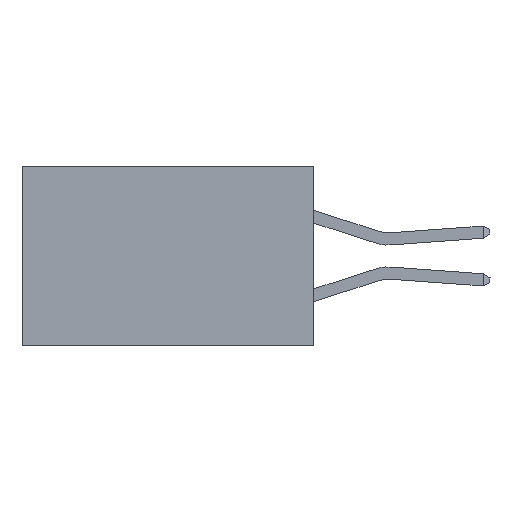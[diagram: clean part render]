
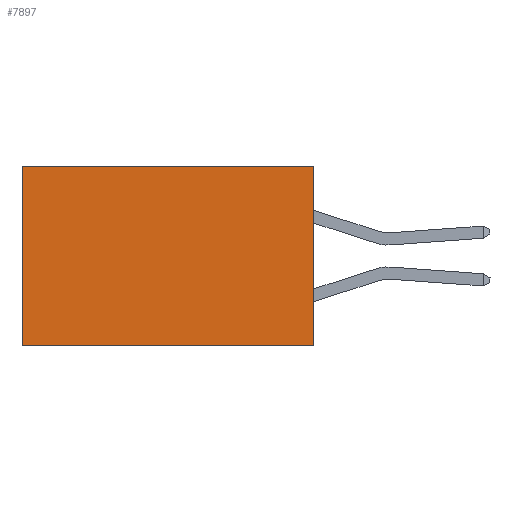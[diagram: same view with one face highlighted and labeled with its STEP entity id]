
A CAD part, left-side view. The second image highlights one B-rep face of the part: STEP entity #7897.
In plain terms, the highlighted planar face has unit normal (-1, 0, 0).
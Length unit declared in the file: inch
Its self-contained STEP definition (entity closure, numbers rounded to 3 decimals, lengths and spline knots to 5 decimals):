
#420 = VECTOR ( 'NONE', #7155, 39.37008 ) ;
#629 = CARTESIAN_POINT ( 'NONE',  ( 0.2875, 0., -0.37 ) ) ;
#686 = VERTEX_POINT ( 'NONE', #1761 ) ;
#1224 = ORIENTED_EDGE ( 'NONE', *, *, #5852, .F. ) ;
#1421 = EDGE_CURVE ( 'NONE', #686, #5934, #5172, .T. ) ;
#1761 = CARTESIAN_POINT ( 'NONE',  ( 0.2875, 0., 0. ) ) ;
#1765 = CARTESIAN_POINT ( 'NONE',  ( 0.2875, 0., 0. ) ) ;
#2211 = CARTESIAN_POINT ( 'NONE',  ( 0.2875, 0.6, -0.37 ) ) ;
#2375 = LINE ( 'NONE', #3022, #420 ) ;
#2548 = ORIENTED_EDGE ( 'NONE', *, *, #4439, .F. ) ;
#2642 = VERTEX_POINT ( 'NONE', #2211 ) ;
#2673 = ORIENTED_EDGE ( 'NONE', *, *, #1421, .T. ) ;
#2735 = AXIS2_PLACEMENT_3D ( 'NONE', #5679, #3637, #8225 ) ;
#2914 = FACE_OUTER_BOUND ( 'NONE', #3984, .T. ) ;
#2983 = PLANE ( 'NONE',  #2735 ) ;
#3022 = CARTESIAN_POINT ( 'NONE',  ( 0.2875, 0., -0.37 ) ) ;
#3075 = VECTOR ( 'NONE', #8655, 39.37008 ) ;
#3130 = CARTESIAN_POINT ( 'NONE',  ( 0.2875, 0.6, 0. ) ) ;
#3423 = ORIENTED_EDGE ( 'NONE', *, *, #3440, .T. ) ;
#3433 = DIRECTION ( 'NONE',  ( 0., 1., 0. ) ) ;
#3440 = EDGE_CURVE ( 'NONE', #5934, #2642, #6630, .T. ) ;
#3637 = DIRECTION ( 'NONE',  ( 1., 0., 0. ) ) ;
#3667 = LINE ( 'NONE', #6379, #5019 ) ;
#3984 = EDGE_LOOP ( 'NONE', ( #3423, #1224, #2548, #2673 ) ) ;
#4439 = EDGE_CURVE ( 'NONE', #686, #5894, #3667, .T. ) ;
#5019 = VECTOR ( 'NONE', #8525, 39.37008 ) ;
#5172 = LINE ( 'NONE', #1765, #6987 ) ;
#5679 = CARTESIAN_POINT ( 'NONE',  ( 0.2875, 0., 0. ) ) ;
#5852 = EDGE_CURVE ( 'NONE', #5894, #2642, #2375, .T. ) ;
#5894 = VERTEX_POINT ( 'NONE', #629 ) ;
#5934 = VERTEX_POINT ( 'NONE', #3130 ) ;
#6134 = CARTESIAN_POINT ( 'NONE',  ( 0.2875, 0.6, 0. ) ) ;
#6379 = CARTESIAN_POINT ( 'NONE',  ( 0.2875, 0., 0. ) ) ;
#6630 = LINE ( 'NONE', #6134, #3075 ) ;
#6987 = VECTOR ( 'NONE', #3433, 39.37008 ) ;
#7155 = DIRECTION ( 'NONE',  ( 0., 1., 0. ) ) ;
#7897 = ADVANCED_FACE ( 'NONE', ( #2914 ), #2983, .F. ) ;
#8225 = DIRECTION ( 'NONE',  ( 0., 0., -1. ) ) ;
#8525 = DIRECTION ( 'NONE',  ( 0., 0., -1. ) ) ;
#8655 = DIRECTION ( 'NONE',  ( 0., 0., -1. ) ) ;
